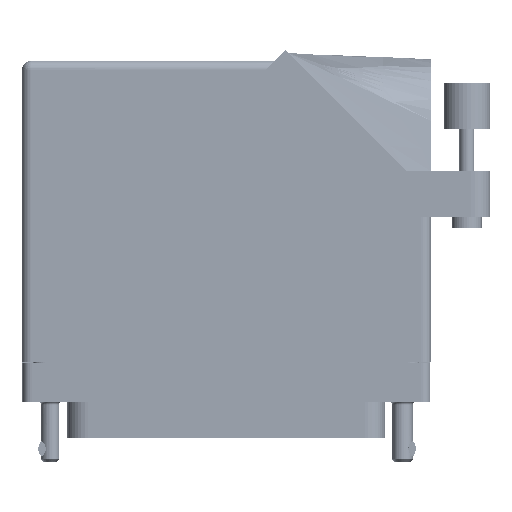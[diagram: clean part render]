
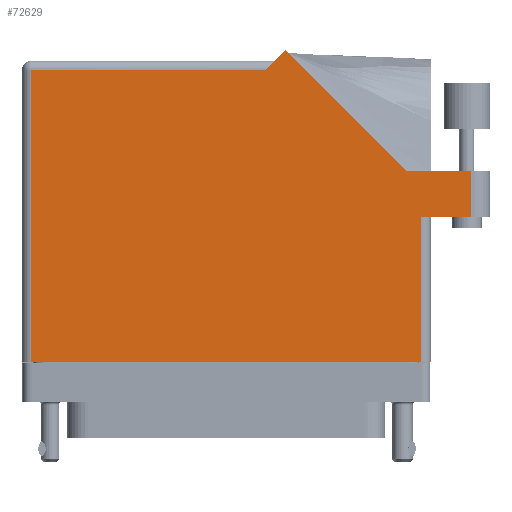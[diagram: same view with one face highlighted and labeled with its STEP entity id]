
A CAD part, front view. The second image highlights one B-rep face of the part: STEP entity #72629.
In plain terms, the highlighted face is planar.
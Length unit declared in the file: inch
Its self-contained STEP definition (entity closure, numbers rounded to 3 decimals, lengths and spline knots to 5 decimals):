
#2840 = CARTESIAN_POINT ( 'NONE',  ( 1.21192, 1.187, 0.765 ) ) ;
#2851 = VECTOR ( 'NONE', #84023, 39.37008 ) ;
#4454 = EDGE_CURVE ( 'NONE', #15791, #16189, #33134, .T. ) ;
#4587 = ORIENTED_EDGE ( 'NONE', *, *, #33388, .T. ) ;
#9800 = ORIENTED_EDGE ( 'NONE', *, *, #71214, .T. ) ;
#10809 = CARTESIAN_POINT ( 'NONE',  ( -1.3775, 1.93, 0.765 ) ) ;
#12339 = VECTOR ( 'NONE', #68902, 39.37008 ) ;
#12346 = DIRECTION ( 'NONE',  ( 1., 0., 0. ) ) ;
#12818 = CARTESIAN_POINT ( 'NONE',  ( 1.21192, 1.187, 0.765 ) ) ;
#14768 = EDGE_CURVE ( 'NONE', #66888, #88118, #46988, .T. ) ;
#15791 = VERTEX_POINT ( 'NONE', #97569 ) ;
#15842 = CARTESIAN_POINT ( 'NONE',  ( -1.3775, 1.868, 0.765 ) ) ;
#16189 = VERTEX_POINT ( 'NONE', #86471 ) ;
#17863 = CARTESIAN_POINT ( 'NONE',  ( 1.3155, 0.88, 0.765 ) ) ;
#20763 = LINE ( 'NONE', #15842, #39472 ) ;
#21480 = EDGE_LOOP ( 'NONE', ( #100741, #65396, #99944, #9800, #4587, #34820, #90962, #53758, #73181 ) ) ;
#27299 = DIRECTION ( 'NONE',  ( 1., 0., 0. ) ) ;
#27736 = EDGE_CURVE ( 'NONE', #30692, #66888, #45074, .T. ) ;
#30055 = VECTOR ( 'NONE', #46024, 39.37008 ) ;
#30692 = VERTEX_POINT ( 'NONE', #17863 ) ;
#30790 = VERTEX_POINT ( 'NONE', #2840 ) ;
#31167 = AXIS2_PLACEMENT_3D ( 'NONE', #10809, #82913, #83249 ) ;
#32228 = LINE ( 'NONE', #58927, #91961 ) ;
#33134 = LINE ( 'NONE', #90336, #44270 ) ;
#33388 = EDGE_CURVE ( 'NONE', #45019, #43706, #82576, .T. ) ;
#34820 = ORIENTED_EDGE ( 'NONE', *, *, #67475, .T. ) ;
#37323 = EDGE_CURVE ( 'NONE', #16189, #30692, #32228, .T. ) ;
#37372 = LINE ( 'NONE', #12818, #12339 ) ;
#39472 = VECTOR ( 'NONE', #48192, 39.37008 ) ;
#43643 = CARTESIAN_POINT ( 'NONE',  ( 1.6525, 1.187, 0.765 ) ) ;
#43706 = VERTEX_POINT ( 'NONE', #79810 ) ;
#44270 = VECTOR ( 'NONE', #12346, 39.37008 ) ;
#45019 = VERTEX_POINT ( 'NONE', #95655 ) ;
#45074 = LINE ( 'NONE', #90221, #102285 ) ;
#45152 = CARTESIAN_POINT ( 'NONE',  ( -1.3155, 1.868, 0.765 ) ) ;
#45278 = LINE ( 'NONE', #60097, #2851 ) ;
#46024 = DIRECTION ( 'NONE',  ( -1., 0., 0. ) ) ;
#46988 = LINE ( 'NONE', #43643, #101713 ) ;
#48192 = DIRECTION ( 'NONE',  ( -1., 0., 0. ) ) ;
#52998 = CARTESIAN_POINT ( 'NONE',  ( 1.7775, 1.187, 0.765 ) ) ;
#53758 = ORIENTED_EDGE ( 'NONE', *, *, #4454, .T. ) ;
#53763 = EDGE_CURVE ( 'NONE', #88118, #30790, #92193, .T. ) ;
#55231 = CARTESIAN_POINT ( 'NONE',  ( 1.6525, 1.187, 0.765 ) ) ;
#58590 = DIRECTION ( 'NONE',  ( 0., 1., 0. ) ) ;
#58927 = CARTESIAN_POINT ( 'NONE',  ( 1.3155, 0.88, 0.765 ) ) ;
#60058 = EDGE_CURVE ( 'NONE', #66570, #15791, #45278, .T. ) ;
#60097 = CARTESIAN_POINT ( 'NONE',  ( -1.3155, -0.1, 0.765 ) ) ;
#65396 = ORIENTED_EDGE ( 'NONE', *, *, #14768, .T. ) ;
#66560 = PLANE ( 'NONE',  #31167 ) ;
#66570 = VERTEX_POINT ( 'NONE', #45152 ) ;
#66888 = VERTEX_POINT ( 'NONE', #93172 ) ;
#67294 = DIRECTION ( 'NONE',  ( 0., 1., 0. ) ) ;
#67475 = EDGE_CURVE ( 'NONE', #43706, #66570, #20763, .T. ) ;
#68902 = DIRECTION ( 'NONE',  ( -0.707, 0.707, 0. ) ) ;
#68929 = VECTOR ( 'NONE', #86740, 39.37008 ) ;
#70405 = CARTESIAN_POINT ( 'NONE',  ( 0.3275, 1.93, 0.765 ) ) ;
#71214 = EDGE_CURVE ( 'NONE', #30790, #45019, #37372, .T. ) ;
#72629 = ADVANCED_FACE ( 'NONE', ( #91957 ), #66560, .F. ) ;
#73181 = ORIENTED_EDGE ( 'NONE', *, *, #37323, .T. ) ;
#79810 = CARTESIAN_POINT ( 'NONE',  ( 0.2655, 1.868, 0.765 ) ) ;
#82576 = LINE ( 'NONE', #70405, #68929 ) ;
#82913 = DIRECTION ( 'NONE',  ( 0., 0., -1. ) ) ;
#83249 = DIRECTION ( 'NONE',  ( -1., 0., 0. ) ) ;
#84023 = DIRECTION ( 'NONE',  ( 0., -1., 0. ) ) ;
#86471 = CARTESIAN_POINT ( 'NONE',  ( 1.3155, -0.1, 0.765 ) ) ;
#86740 = DIRECTION ( 'NONE',  ( -0.707, -0.707, 0. ) ) ;
#88118 = VERTEX_POINT ( 'NONE', #55231 ) ;
#90221 = CARTESIAN_POINT ( 'NONE',  ( 1.3775, 0.88, 0.765 ) ) ;
#90336 = CARTESIAN_POINT ( 'NONE',  ( -1.3775, -0.1, 0.765 ) ) ;
#90962 = ORIENTED_EDGE ( 'NONE', *, *, #60058, .T. ) ;
#91957 = FACE_OUTER_BOUND ( 'NONE', #21480, .T. ) ;
#91961 = VECTOR ( 'NONE', #58590, 39.37008 ) ;
#92193 = LINE ( 'NONE', #52998, #30055 ) ;
#93172 = CARTESIAN_POINT ( 'NONE',  ( 1.6525, 0.88, 0.765 ) ) ;
#95655 = CARTESIAN_POINT ( 'NONE',  ( 0.39821, 2.00071, 0.765 ) ) ;
#97569 = CARTESIAN_POINT ( 'NONE',  ( -1.3155, -0.1, 0.765 ) ) ;
#99944 = ORIENTED_EDGE ( 'NONE', *, *, #53763, .T. ) ;
#100741 = ORIENTED_EDGE ( 'NONE', *, *, #27736, .T. ) ;
#101713 = VECTOR ( 'NONE', #67294, 39.37008 ) ;
#102285 = VECTOR ( 'NONE', #27299, 39.37008 ) ;
